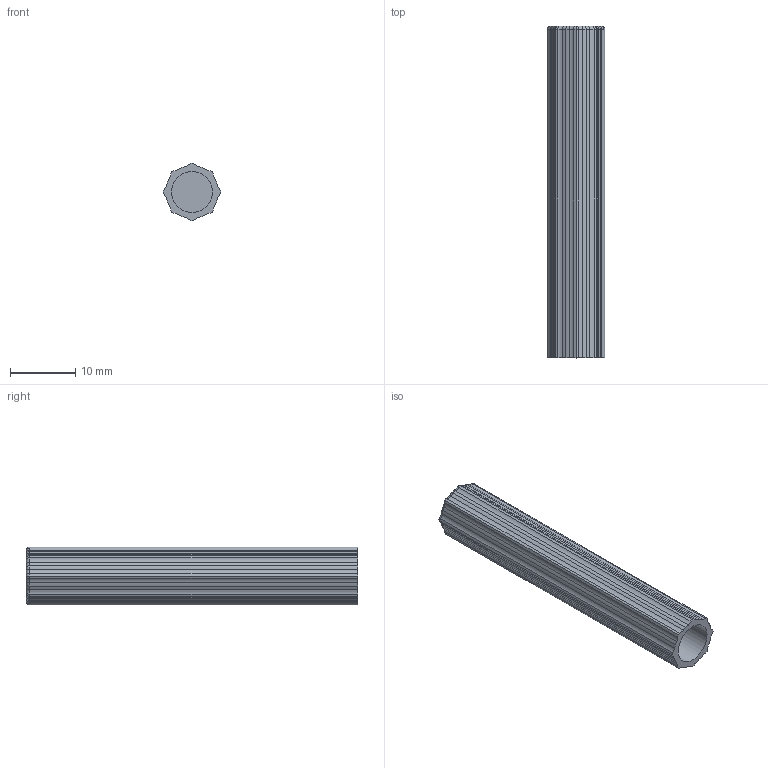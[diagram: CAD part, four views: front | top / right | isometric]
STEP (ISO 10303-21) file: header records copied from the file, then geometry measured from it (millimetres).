
FILE_DESCRIPTION(/* description */ (''),/* implementation_level */ '2;1');
FILE_NAME(/* name */ 'Chambering Insulator Metric (6mm).stp',/* time_stamp */ '2021-02-15T01:39:57-06:00',/* author */ ('johne'),/* organization */ (''),/* preprocessor_version */ 'ST-DEVELOPER v18',/* originating_system */ 'Autodesk Inventor 2020',/* authorisation */ '');
FILE_SCHEMA (('AUTOMOTIVE_DESIGN { 1 0 10303 214 3 1 1 }'));
Length unit declared in the file: millimetre
Products named in the file (1): Chambering Insulator 6mm rod
Bounding box: 8.82 x 50.8 x 8.82 mm (x, y, z)
Volume: 1234.5 mm3; surface area: 2435.7 mm2
Topology: 1 solids, 1 shells, 100 faces, 259 edges, 162 vertices
Faces by surface type: cylinder 49, torus 32, plane 19
Full cylindrical faces by diameter (mm): 6.25 x1
Entity records: 3510 total; most frequent: CARTESIAN_POINT 970, DIRECTION 559, ORIENTED_EDGE 518, EDGE_CURVE 259, AXIS2_PLACEMENT_3D 223, VERTEX_POINT 162, CIRCLE 114, LINE 113
